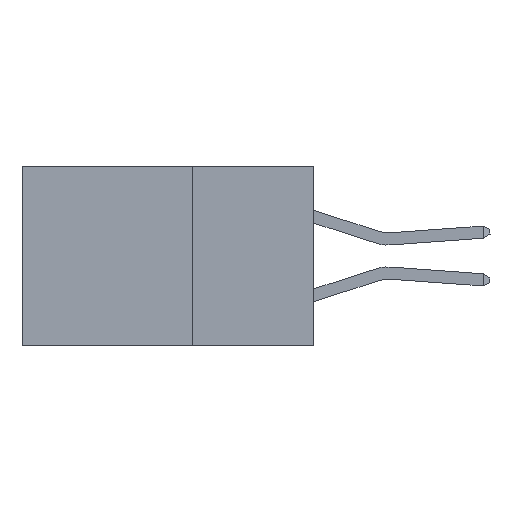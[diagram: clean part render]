
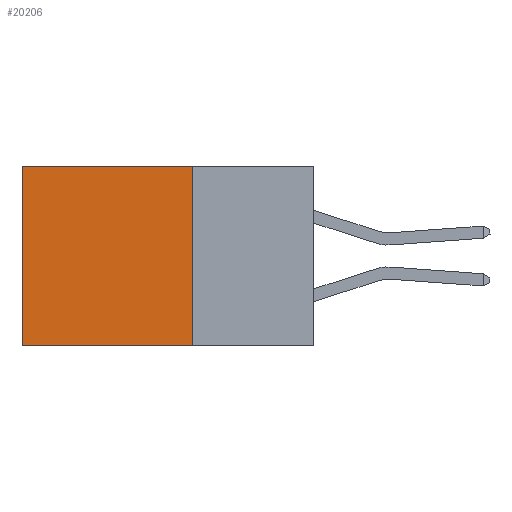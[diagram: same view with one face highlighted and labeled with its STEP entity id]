
A CAD part, left-side view. The second image highlights one B-rep face of the part: STEP entity #20206.
In plain terms, the highlighted planar face has unit normal (-1, 0, 0).
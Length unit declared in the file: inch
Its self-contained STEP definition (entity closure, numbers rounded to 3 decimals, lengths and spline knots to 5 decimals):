
#1299 = CARTESIAN_POINT ( 'NONE',  ( 0.2875, 0.25, 0. ) ) ;
#1597 = VERTEX_POINT ( 'NONE', #12496 ) ;
#2142 = VECTOR ( 'NONE', #9279, 39.37008 ) ;
#2870 = PLANE ( 'NONE',  #10201 ) ;
#4509 = CARTESIAN_POINT ( 'NONE',  ( 0.2875, 0.25, 0. ) ) ;
#5380 = EDGE_CURVE ( 'NONE', #1597, #9938, #9385, .T. ) ;
#5511 = EDGE_LOOP ( 'NONE', ( #11576, #15126, #18954, #12999 ) ) ;
#6165 = CARTESIAN_POINT ( 'NONE',  ( 0.2875, 0.25, 0. ) ) ;
#7527 = CARTESIAN_POINT ( 'NONE',  ( 0.2875, 0.6, 0. ) ) ;
#7946 = VERTEX_POINT ( 'NONE', #4509 ) ;
#8005 = DIRECTION ( 'NONE',  ( 0., 1., 0. ) ) ;
#8543 = DIRECTION ( 'NONE',  ( 0., 1., 0. ) ) ;
#8788 = VECTOR ( 'NONE', #8543, 39.37008 ) ;
#9279 = DIRECTION ( 'NONE',  ( 0., 0., -1. ) ) ;
#9385 = LINE ( 'NONE', #7527, #18218 ) ;
#9938 = VERTEX_POINT ( 'NONE', #15146 ) ;
#10201 = AXIS2_PLACEMENT_3D ( 'NONE', #1299, #18213, #13451 ) ;
#11040 = LINE ( 'NONE', #6165, #2142 ) ;
#11356 = LINE ( 'NONE', #13407, #8788 ) ;
#11576 = ORIENTED_EDGE ( 'NONE', *, *, #5380, .T. ) ;
#11604 = EDGE_CURVE ( 'NONE', #11982, #9938, #19097, .T. ) ;
#11982 = VERTEX_POINT ( 'NONE', #14411 ) ;
#12496 = CARTESIAN_POINT ( 'NONE',  ( 0.2875, 0.6, 0. ) ) ;
#12673 = CARTESIAN_POINT ( 'NONE',  ( 0.2875, 0.25, -0.37 ) ) ;
#12999 = ORIENTED_EDGE ( 'NONE', *, *, #15594, .T. ) ;
#13407 = CARTESIAN_POINT ( 'NONE',  ( 0.2875, 0.25, 0. ) ) ;
#13451 = DIRECTION ( 'NONE',  ( 0., 0., -1. ) ) ;
#14411 = CARTESIAN_POINT ( 'NONE',  ( 0.2875, 0.25, -0.37 ) ) ;
#15126 = ORIENTED_EDGE ( 'NONE', *, *, #11604, .F. ) ;
#15146 = CARTESIAN_POINT ( 'NONE',  ( 0.2875, 0.6, -0.37 ) ) ;
#15492 = EDGE_CURVE ( 'NONE', #7946, #11982, #11040, .T. ) ;
#15594 = EDGE_CURVE ( 'NONE', #7946, #1597, #11356, .T. ) ;
#17055 = DIRECTION ( 'NONE',  ( 0., 0., -1. ) ) ;
#17072 = FACE_OUTER_BOUND ( 'NONE', #5511, .T. ) ;
#18213 = DIRECTION ( 'NONE',  ( 1., 0., 0. ) ) ;
#18218 = VECTOR ( 'NONE', #17055, 39.37008 ) ;
#18954 = ORIENTED_EDGE ( 'NONE', *, *, #15492, .F. ) ;
#19097 = LINE ( 'NONE', #12673, #20254 ) ;
#20206 = ADVANCED_FACE ( 'NONE', ( #17072 ), #2870, .F. ) ;
#20254 = VECTOR ( 'NONE', #8005, 39.37008 ) ;
